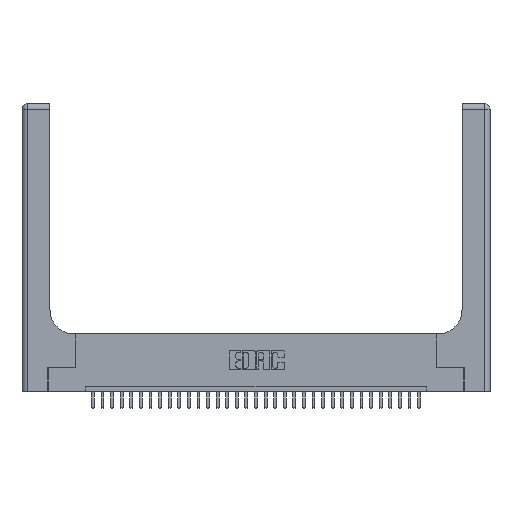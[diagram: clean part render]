
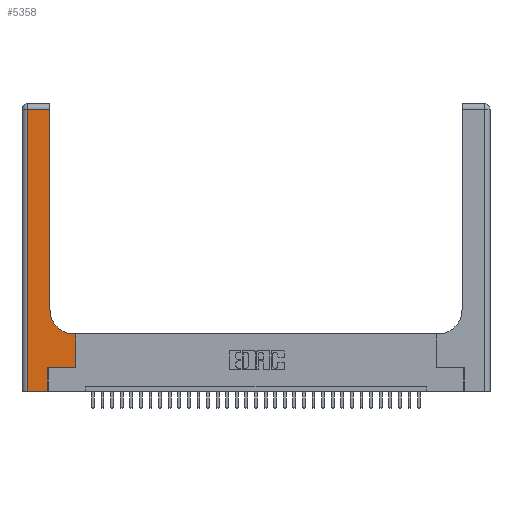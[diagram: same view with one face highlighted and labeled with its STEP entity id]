
A CAD part, top view. The second image highlights one B-rep face of the part: STEP entity #5358.
In plain terms, the highlighted planar face has unit normal (0, 0, 1).
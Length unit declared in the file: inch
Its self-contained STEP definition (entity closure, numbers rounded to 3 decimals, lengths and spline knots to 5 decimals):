
#96 = VECTOR ( 'NONE', #32562, 39.37008 ) ;
#539 = DIRECTION ( 'NONE',  ( 1., 0., 0. ) ) ;
#758 = EDGE_CURVE ( 'NONE', #19674, #24998, #11797, .T. ) ;
#1579 = ORIENTED_EDGE ( 'NONE', *, *, #28837, .T. ) ;
#1599 = CARTESIAN_POINT ( 'NONE',  ( 0.06, 2.94, 0.37 ) ) ;
#1866 = DIRECTION ( 'NONE',  ( 0., 0., -1. ) ) ;
#2083 = PLANE ( 'NONE',  #18109 ) ;
#2491 = EDGE_CURVE ( 'NONE', #15856, #22832, #29441, .T. ) ;
#2584 = LINE ( 'NONE', #20098, #17904 ) ;
#2679 = ORIENTED_EDGE ( 'NONE', *, *, #25447, .T. ) ;
#3123 = ORIENTED_EDGE ( 'NONE', *, *, #15527, .T. ) ;
#4031 = DIRECTION ( 'NONE',  ( 0., 1., 0. ) ) ;
#5358 = ADVANCED_FACE ( 'NONE', ( #24328 ), #2083, .F. ) ;
#5707 = LINE ( 'NONE', #14648, #29682 ) ;
#6426 = CARTESIAN_POINT ( 'NONE',  ( 0.5415, 0.85, 0.37 ) ) ;
#6949 = LINE ( 'NONE', #13038, #21879 ) ;
#7112 = CARTESIAN_POINT ( 'NONE',  ( 0.5585, 0.6, 0.37 ) ) ;
#7512 = CARTESIAN_POINT ( 'NONE',  ( 0.269, 0.25, 0.37 ) ) ;
#7775 = CARTESIAN_POINT ( 'NONE',  ( 0.2915, 0.6, 0.37 ) ) ;
#8173 = ORIENTED_EDGE ( 'NONE', *, *, #22554, .T. ) ;
#8420 = VERTEX_POINT ( 'NONE', #14344 ) ;
#9253 = DIRECTION ( 'NONE',  ( 0., 1., 0. ) ) ;
#9263 = ORIENTED_EDGE ( 'NONE', *, *, #2491, .T. ) ;
#9282 = VERTEX_POINT ( 'NONE', #7512 ) ;
#10843 = ORIENTED_EDGE ( 'NONE', *, *, #758, .T. ) ;
#11432 = VECTOR ( 'NONE', #27986, 39.37008 ) ;
#11797 = LINE ( 'NONE', #19044, #29506 ) ;
#11958 = EDGE_LOOP ( 'NONE', ( #10843, #2679, #21326, #3123, #8173, #1579, #18714, #9263, #19642 ) ) ;
#12462 = DIRECTION ( 'NONE',  ( 1., 0., 0. ) ) ;
#12598 = CARTESIAN_POINT ( 'NONE',  ( 0.5585, 0.25, 0.37 ) ) ;
#13038 = CARTESIAN_POINT ( 'NONE',  ( 0., 0., 0.37 ) ) ;
#14195 = VERTEX_POINT ( 'NONE', #25654 ) ;
#14344 = CARTESIAN_POINT ( 'NONE',  ( 0.5585, 0.25, 0.37 ) ) ;
#14469 = VERTEX_POINT ( 'NONE', #1599 ) ;
#14552 = EDGE_CURVE ( 'NONE', #22832, #19674, #19543, .T. ) ;
#14648 = CARTESIAN_POINT ( 'NONE',  ( 0.269, 0., 0.37 ) ) ;
#15527 = EDGE_CURVE ( 'NONE', #14195, #16547, #6949, .T. ) ;
#15856 = VERTEX_POINT ( 'NONE', #7112 ) ;
#16547 = VERTEX_POINT ( 'NONE', #20019 ) ;
#17307 = VECTOR ( 'NONE', #12462, 39.37008 ) ;
#17904 = VECTOR ( 'NONE', #19998, 39.37008 ) ;
#18109 = AXIS2_PLACEMENT_3D ( 'NONE', #24673, #1866, #32064 ) ;
#18714 = ORIENTED_EDGE ( 'NONE', *, *, #28279, .T. ) ;
#19044 = CARTESIAN_POINT ( 'NONE',  ( 0.2915, 3., 0.37 ) ) ;
#19543 = CIRCLE ( 'NONE', #26666, 0.25 ) ;
#19640 = CARTESIAN_POINT ( 'NONE',  ( 0.2915, 0.85, 0.37 ) ) ;
#19642 = ORIENTED_EDGE ( 'NONE', *, *, #14552, .T. ) ;
#19671 = LINE ( 'NONE', #19940, #17307 ) ;
#19674 = VERTEX_POINT ( 'NONE', #19640 ) ;
#19940 = CARTESIAN_POINT ( 'NONE',  ( 0.269, 0.25, 0.37 ) ) ;
#19998 = DIRECTION ( 'NONE',  ( -1., 0., 0. ) ) ;
#20019 = CARTESIAN_POINT ( 'NONE',  ( 0.269, 0., 0.37 ) ) ;
#20088 = DIRECTION ( 'NONE',  ( -1., 0., 0. ) ) ;
#20098 = CARTESIAN_POINT ( 'NONE',  ( 0., 2.94, 0.37 ) ) ;
#21326 = ORIENTED_EDGE ( 'NONE', *, *, #30748, .T. ) ;
#21480 = DIRECTION ( 'NONE',  ( 0., 0., -1. ) ) ;
#21879 = VECTOR ( 'NONE', #539, 39.37008 ) ;
#22554 = EDGE_CURVE ( 'NONE', #16547, #9282, #5707, .T. ) ;
#22832 = VERTEX_POINT ( 'NONE', #28060 ) ;
#23993 = DIRECTION ( 'NONE',  ( 1., 0., 0. ) ) ;
#24328 = FACE_OUTER_BOUND ( 'NONE', #11958, .T. ) ;
#24673 = CARTESIAN_POINT ( 'NONE',  ( 0., 3., 0.37 ) ) ;
#24998 = VERTEX_POINT ( 'NONE', #30788 ) ;
#25447 = EDGE_CURVE ( 'NONE', #24998, #14469, #2584, .T. ) ;
#25654 = CARTESIAN_POINT ( 'NONE',  ( 0.06, 0., 0.37 ) ) ;
#26666 = AXIS2_PLACEMENT_3D ( 'NONE', #6426, #21480, #23993 ) ;
#27244 = LINE ( 'NONE', #32460, #96 ) ;
#27986 = DIRECTION ( 'NONE',  ( 0., 1., 0. ) ) ;
#28060 = CARTESIAN_POINT ( 'NONE',  ( 0.5415, 0.6, 0.37 ) ) ;
#28279 = EDGE_CURVE ( 'NONE', #8420, #15856, #29151, .T. ) ;
#28837 = EDGE_CURVE ( 'NONE', #9282, #8420, #19671, .T. ) ;
#29151 = LINE ( 'NONE', #12598, #11432 ) ;
#29441 = LINE ( 'NONE', #7775, #30621 ) ;
#29506 = VECTOR ( 'NONE', #4031, 39.37008 ) ;
#29682 = VECTOR ( 'NONE', #9253, 39.37008 ) ;
#30621 = VECTOR ( 'NONE', #20088, 39.37008 ) ;
#30748 = EDGE_CURVE ( 'NONE', #14469, #14195, #27244, .T. ) ;
#30788 = CARTESIAN_POINT ( 'NONE',  ( 0.2915, 2.94, 0.37 ) ) ;
#32064 = DIRECTION ( 'NONE',  ( -1., 0., 0. ) ) ;
#32460 = CARTESIAN_POINT ( 'NONE',  ( 0.06, 3., 0.37 ) ) ;
#32562 = DIRECTION ( 'NONE',  ( 0., -1., 0. ) ) ;
